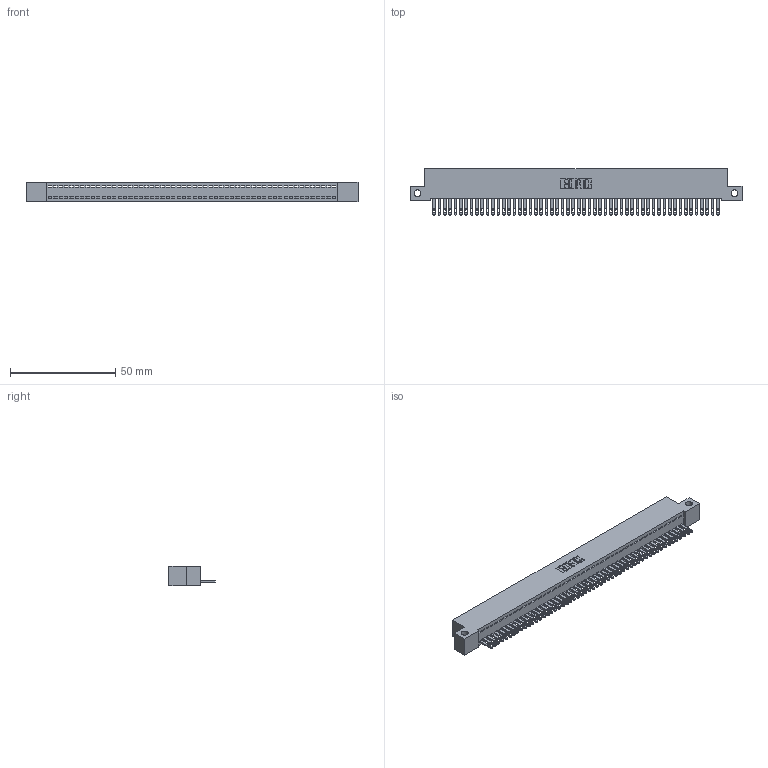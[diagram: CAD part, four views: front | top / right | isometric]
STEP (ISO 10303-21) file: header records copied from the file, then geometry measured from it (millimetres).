
FILE_DESCRIPTION (( 'STEP AP203' ), '1' );
FILE_NAME ('342-054-500-112.STEP', '2019-10-03T02:35:24', ( '' ), ( '' ), 'SwSTEP 2.0', 'SolidWorks 2016', '' );
FILE_SCHEMA (( 'CONFIG_CONTROL_DESIGN' ));
Length unit declared in the file: inch
Products named in the file (3): 342-054-500-112; 342 Part_Side Mount; 345-292-001_345-293-100
Assembly tree (55 placements, depth 2):
  342-054-500-112
    342 Part_Side Mount
    345-292-001_345-293-100  x54
Bounding box: 157.48 x 21.85 x 9.4 mm (x, y, z)
Volume: 13811.5 mm3; surface area: 20448.9 mm2
Topology: 55 solids, 55 shells, 3026 faces, 9371 edges, 6246 vertices
Faces by surface type: plane 2010, cylinder 1016
Entity records: 31261 total; most frequent: CARTESIAN_POINT 5396, ORIENTED_EDGE 5386, DIRECTION 4529, EDGE_CURVE 2693, VECTOR 2561, LINE 2561, VERTEX_POINT 1794, AXIS2_PLACEMENT_3D 984
